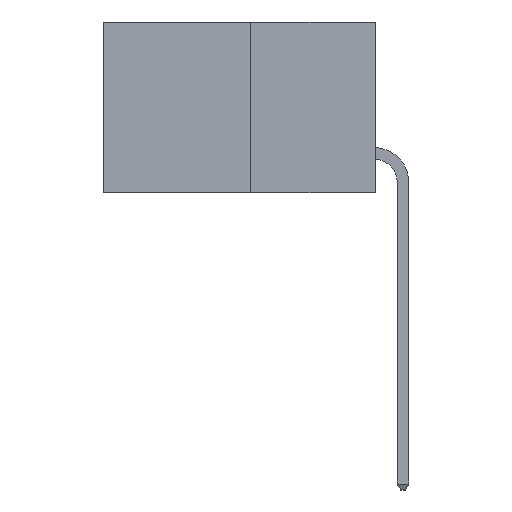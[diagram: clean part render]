
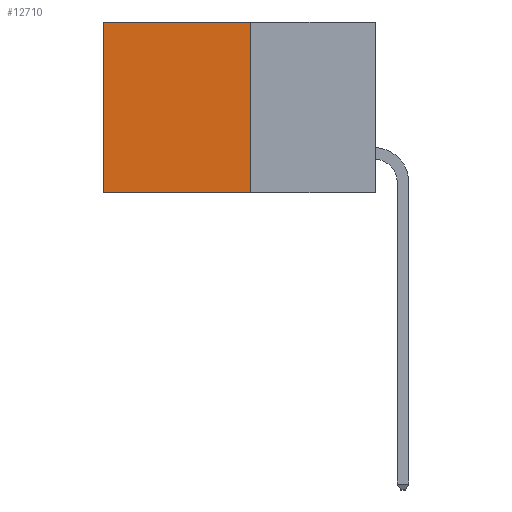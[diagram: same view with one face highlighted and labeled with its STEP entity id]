
A CAD part, left-side view. The second image highlights one B-rep face of the part: STEP entity #12710.
In plain terms, the highlighted planar face has unit normal (-1, 0, 0).
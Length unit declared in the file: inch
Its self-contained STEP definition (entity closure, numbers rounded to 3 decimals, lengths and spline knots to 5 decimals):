
#260 = DIRECTION ( 'NONE',  ( 1., 0., 0. ) ) ;
#406 = EDGE_CURVE ( 'NONE', #9822, #4685, #8190, .T. ) ;
#976 = CARTESIAN_POINT ( 'NONE',  ( 0.277, 0.27, 0. ) ) ;
#1540 = VECTOR ( 'NONE', #11101, 39.37008 ) ;
#1567 = VECTOR ( 'NONE', #7884, 39.37008 ) ;
#2466 = DIRECTION ( 'NONE',  ( 0., 0., -1. ) ) ;
#2609 = EDGE_CURVE ( 'NONE', #9822, #10539, #14812, .T. ) ;
#4403 = ORIENTED_EDGE ( 'NONE', *, *, #8375, .F. ) ;
#4685 = VERTEX_POINT ( 'NONE', #10964 ) ;
#4887 = LINE ( 'NONE', #9904, #1540 ) ;
#5472 = VERTEX_POINT ( 'NONE', #12205 ) ;
#5636 = DIRECTION ( 'NONE',  ( 0., 1., 0. ) ) ;
#6129 = LINE ( 'NONE', #11653, #9001 ) ;
#7115 = AXIS2_PLACEMENT_3D ( 'NONE', #12450, #260, #8927 ) ;
#7733 = PLANE ( 'NONE',  #7115 ) ;
#7884 = DIRECTION ( 'NONE',  ( 0., 1., 0. ) ) ;
#8190 = LINE ( 'NONE', #10775, #1567 ) ;
#8375 = EDGE_CURVE ( 'NONE', #10539, #5472, #6129, .T. ) ;
#8927 = DIRECTION ( 'NONE',  ( 0., 0., -1. ) ) ;
#9001 = VECTOR ( 'NONE', #5636, 39.37008 ) ;
#9489 = FACE_OUTER_BOUND ( 'NONE', #14263, .T. ) ;
#9814 = CARTESIAN_POINT ( 'NONE',  ( 0.277, 0.27, -0.37 ) ) ;
#9822 = VERTEX_POINT ( 'NONE', #976 ) ;
#9900 = ORIENTED_EDGE ( 'NONE', *, *, #406, .T. ) ;
#9904 = CARTESIAN_POINT ( 'NONE',  ( 0.277, 0.59, -0.37 ) ) ;
#10047 = ORIENTED_EDGE ( 'NONE', *, *, #2609, .F. ) ;
#10539 = VERTEX_POINT ( 'NONE', #9814 ) ;
#10564 = ORIENTED_EDGE ( 'NONE', *, *, #11277, .T. ) ;
#10775 = CARTESIAN_POINT ( 'NONE',  ( 0.277, 0.27, 0. ) ) ;
#10964 = CARTESIAN_POINT ( 'NONE',  ( 0.277, 0.59, 0. ) ) ;
#11101 = DIRECTION ( 'NONE',  ( 0., 0., -1. ) ) ;
#11277 = EDGE_CURVE ( 'NONE', #4685, #5472, #4887, .T. ) ;
#11288 = VECTOR ( 'NONE', #2466, 39.37008 ) ;
#11653 = CARTESIAN_POINT ( 'NONE',  ( 0.277, 0.27, -0.37 ) ) ;
#12205 = CARTESIAN_POINT ( 'NONE',  ( 0.277, 0.59, -0.37 ) ) ;
#12450 = CARTESIAN_POINT ( 'NONE',  ( 0.277, 0.27, -0.37 ) ) ;
#12710 = ADVANCED_FACE ( 'NONE', ( #9489 ), #7733, .F. ) ;
#14263 = EDGE_LOOP ( 'NONE', ( #10564, #4403, #10047, #9900 ) ) ;
#14696 = CARTESIAN_POINT ( 'NONE',  ( 0.277, 0.27, -0.37 ) ) ;
#14812 = LINE ( 'NONE', #14696, #11288 ) ;
